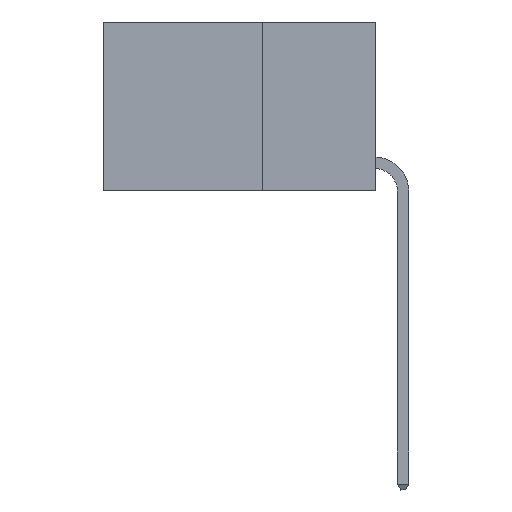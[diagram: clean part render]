
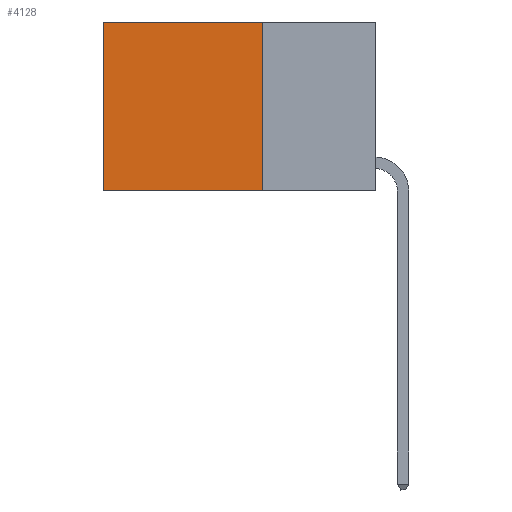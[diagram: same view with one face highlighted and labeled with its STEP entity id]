
A CAD part, left-side view. The second image highlights one B-rep face of the part: STEP entity #4128.
In plain terms, the highlighted planar face has unit normal (-1, 0, 0).
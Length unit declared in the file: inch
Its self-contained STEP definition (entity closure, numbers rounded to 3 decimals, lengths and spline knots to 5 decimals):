
#1425 = EDGE_CURVE ( 'NONE', #4784, #4338, #5465, .T. ) ;
#2165 = ORIENTED_EDGE ( 'NONE', *, *, #7312, .F. ) ;
#3617 = LINE ( 'NONE', #4743, #4047 ) ;
#3855 = FACE_OUTER_BOUND ( 'NONE', #5369, .T. ) ;
#4047 = VECTOR ( 'NONE', #16514, 39.37008 ) ;
#4120 = DIRECTION ( 'NONE',  ( 0., 0., -1. ) ) ;
#4128 = ADVANCED_FACE ( 'NONE', ( #3855 ), #14349, .F. ) ;
#4338 = VERTEX_POINT ( 'NONE', #4705 ) ;
#4569 = DIRECTION ( 'NONE',  ( 0., 0., -1. ) ) ;
#4705 = CARTESIAN_POINT ( 'NONE',  ( 0.2625, 0.6, -0.37 ) ) ;
#4743 = CARTESIAN_POINT ( 'NONE',  ( 0.2625, 0.25, -0.37 ) ) ;
#4784 = VERTEX_POINT ( 'NONE', #10205 ) ;
#5369 = EDGE_LOOP ( 'NONE', ( #11678, #2165, #6004, #16457 ) ) ;
#5465 = LINE ( 'NONE', #9363, #15441 ) ;
#5859 = LINE ( 'NONE', #16266, #13572 ) ;
#6004 = ORIENTED_EDGE ( 'NONE', *, *, #7310, .F. ) ;
#7310 = EDGE_CURVE ( 'NONE', #8832, #16123, #5859, .T. ) ;
#7312 = EDGE_CURVE ( 'NONE', #16123, #4338, #3617, .T. ) ;
#7850 = DIRECTION ( 'NONE',  ( 0., 1., 0. ) ) ;
#8708 = CARTESIAN_POINT ( 'NONE',  ( 0.2625, 0.25, 0. ) ) ;
#8832 = VERTEX_POINT ( 'NONE', #8708 ) ;
#9363 = CARTESIAN_POINT ( 'NONE',  ( 0.2625, 0.6, 0. ) ) ;
#10205 = CARTESIAN_POINT ( 'NONE',  ( 0.2625, 0.6, 0. ) ) ;
#10330 = EDGE_CURVE ( 'NONE', #8832, #4784, #13321, .T. ) ;
#10507 = DIRECTION ( 'NONE',  ( 1., 0., 0. ) ) ;
#10826 = AXIS2_PLACEMENT_3D ( 'NONE', #11686, #10507, #4120 ) ;
#11678 = ORIENTED_EDGE ( 'NONE', *, *, #1425, .T. ) ;
#11686 = CARTESIAN_POINT ( 'NONE',  ( 0.2625, 0.25, 0. ) ) ;
#12010 = CARTESIAN_POINT ( 'NONE',  ( 0.2625, 0.25, 0. ) ) ;
#13321 = LINE ( 'NONE', #12010, #14977 ) ;
#13388 = DIRECTION ( 'NONE',  ( 0., 0., -1. ) ) ;
#13572 = VECTOR ( 'NONE', #4569, 39.37008 ) ;
#14349 = PLANE ( 'NONE',  #10826 ) ;
#14977 = VECTOR ( 'NONE', #7850, 39.37008 ) ;
#15441 = VECTOR ( 'NONE', #13388, 39.37008 ) ;
#16123 = VERTEX_POINT ( 'NONE', #16317 ) ;
#16266 = CARTESIAN_POINT ( 'NONE',  ( 0.2625, 0.25, 0. ) ) ;
#16317 = CARTESIAN_POINT ( 'NONE',  ( 0.2625, 0.25, -0.37 ) ) ;
#16457 = ORIENTED_EDGE ( 'NONE', *, *, #10330, .T. ) ;
#16514 = DIRECTION ( 'NONE',  ( 0., 1., 0. ) ) ;
